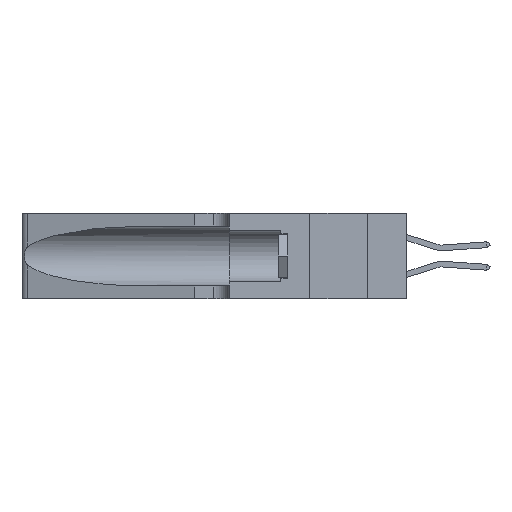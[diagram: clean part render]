
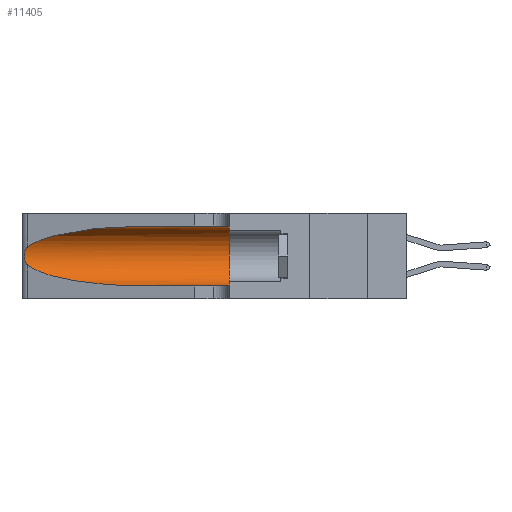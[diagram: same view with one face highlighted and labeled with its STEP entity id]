
A CAD part, left-side view. The second image highlights one B-rep face of the part: STEP entity #11405.
In plain terms, the highlighted cylindrical face has radius 3.308 mm (diameter 6.617 mm), a partial arc.
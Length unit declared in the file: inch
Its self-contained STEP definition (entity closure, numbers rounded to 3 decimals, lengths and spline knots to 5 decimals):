
#397 = CARTESIAN_POINT ( 'NONE',  ( 0.25789, 1.23486, 0.15765 ) ) ;
#1251 = DIRECTION ( 'NONE',  ( 0., -1., 0. ) ) ;
#2952 = CYLINDRICAL_SURFACE ( 'NONE', #24174, 0.13025 ) ;
#3356 = EDGE_CURVE ( 'NONE', #25811, #12666, #20754, .T. ) ;
#3742 = ORIENTED_EDGE ( 'NONE', *, *, #9370, .T. ) ;
#4027 = CARTESIAN_POINT ( 'NONE',  ( 0.18966, 0.96281, 0.31525 ) ) ;
#4162 = ORIENTED_EDGE ( 'NONE', *, *, #6636, .F. ) ;
#4529 = VERTEX_POINT ( 'NONE', #6289 ) ;
#5120 = CARTESIAN_POINT ( 'NONE',  ( 0.26075, 1.23896, 0.178 ) ) ;
#5314 = CARTESIAN_POINT ( 'NONE',  ( 0.25856, 1.23593, 0.16098 ) ) ;
#5771 = CARTESIAN_POINT ( 'NONE',  ( 0.1305, 1.61858, 0.185 ) ) ;
#6289 = CARTESIAN_POINT ( 'NONE',  ( 0.1305, 0.35, 0.05475 ) ) ;
#6322 = CARTESIAN_POINT ( 'NONE',  ( 0.2373, 1.15595, 0.28018 ) ) ;
#6623 = CARTESIAN_POINT ( 'NONE',  ( 0.25487, 1.22718, 0.22369 ) ) ;
#6636 = EDGE_CURVE ( 'NONE', #12883, #4529, #18485, .T. ) ;
#6882 = ORIENTED_EDGE ( 'NONE', *, *, #22389, .T. ) ;
#7833 = CARTESIAN_POINT ( 'NONE',  ( 0.25487, 1.22718, 0.14631 ) ) ;
#7922 = CARTESIAN_POINT ( 'NONE',  ( 0.1305, 1.61858, 0.05475 ) ) ;
#8382 = ORIENTED_EDGE ( 'NONE', *, *, #3356, .T. ) ;
#8412 = VECTOR ( 'NONE', #28521, 39.37008 ) ;
#8670 = CARTESIAN_POINT ( 'NONE',  ( 0.1305, 0.35, 0.31525 ) ) ;
#9370 = EDGE_CURVE ( 'NONE', #22631, #17043, #26556, .T. ) ;
#9446 = DIRECTION ( 'NONE',  ( 0., -1., 0. ) ) ;
#9896 = CARTESIAN_POINT ( 'NONE',  ( 0.25639, 1.23186, 0.15144 ) ) ;
#11096 = DIRECTION ( 'NONE',  ( 0., 0., 1. ) ) ;
#11405 = ADVANCED_FACE ( 'NONE', ( #11924 ), #2952, .F. ) ;
#11717 = CARTESIAN_POINT ( 'NONE',  ( 0.1305, 0.72297, 0.05475 ) ) ;
#11924 = FACE_OUTER_BOUND ( 'NONE', #18745, .T. ) ;
#12104 = CARTESIAN_POINT ( 'NONE',  ( 0.25555, 1.22994, 0.2215 ) ) ;
#12279 = ORIENTED_EDGE ( 'NONE', *, *, #28177, .F. ) ;
#12666 = VERTEX_POINT ( 'NONE', #18245 ) ;
#12883 = VERTEX_POINT ( 'NONE', #8670 ) ;
#13277 = B_SPLINE_CURVE_WITH_KNOTS ( 'NONE', 3,
 ( #14504, #12104, #23615, #27709, #18791, #14099, #18982, #5120, #14199, #5314, #397, #9896, #21247, #19078 ),
 .UNSPECIFIED., .F., .F.,
 ( 4, 2, 2, 2, 2, 2, 4 ),
 ( 0., 0.00027, 0.00053, 0.00107, 0.0016, 0.00187, 0.00214 ),
 .UNSPECIFIED. ) ;
#14099 = CARTESIAN_POINT ( 'NONE',  ( 0.26018, 1.23835, 0.19895 ) ) ;
#14199 = CARTESIAN_POINT ( 'NONE',  ( 0.26017, 1.23833, 0.17102 ) ) ;
#14233 = ORIENTED_EDGE ( 'NONE', *, *, #18139, .T. ) ;
#14504 = CARTESIAN_POINT ( 'NONE',  ( 0.25487, 1.22718, 0.22369 ) ) ;
#15575 = LINE ( 'NONE', #7922, #8412 ) ;
#15642 = CARTESIAN_POINT ( 'NONE',  ( 0.2373, 1.15595, 0.08982 ) ) ;
#17043 = VERTEX_POINT ( 'NONE', #28940 ) ;
#17242 = DIRECTION ( 'NONE',  ( 0., 0., -1. ) ) ;
#18139 = EDGE_CURVE ( 'NONE', #17043, #25811, #13277, .T. ) ;
#18245 = CARTESIAN_POINT ( 'NONE',  ( 0.1305, 0.72297, 0.05475 ) ) ;
#18485 = CIRCLE ( 'NONE', #19364, 0.13025 ) ;
#18745 = EDGE_LOOP ( 'NONE', ( #3742, #14233, #8382, #6882, #4162, #12279 ) ) ;
#18791 = CARTESIAN_POINT ( 'NONE',  ( 0.25854, 1.2359, 0.20912 ) ) ;
#18982 = CARTESIAN_POINT ( 'NONE',  ( 0.26075, 1.23896, 0.19203 ) ) ;
#19078 = CARTESIAN_POINT ( 'NONE',  ( 0.25487, 1.22718, 0.14631 ) ) ;
#19364 = AXIS2_PLACEMENT_3D ( 'NONE', #24706, #22613, #11096 ) ;
#19574 = VECTOR ( 'NONE', #9446, 39.37008 ) ;
#20109 = CARTESIAN_POINT ( 'NONE',  ( 0.1305, 0.72297, 0.31525 ) ) ;
#20700 = CARTESIAN_POINT ( 'NONE',  ( 0.18966, 0.96281, 0.05475 ) ) ;
#20754 =( BOUNDED_CURVE ( )  B_SPLINE_CURVE ( 3, ( #24887, #15642, #20700, #11717 ),
 .UNSPECIFIED., .F., .F. ) 
 B_SPLINE_CURVE_WITH_KNOTS ( ( 4, 4 ),
 ( 3.44316, 4.71239 ),
 .UNSPECIFIED. ) 
 CURVE ( )  GEOMETRIC_REPRESENTATION_ITEM ( )  RATIONAL_B_SPLINE_CURVE ( ( 1., 0.87, 0.87, 1. ) ) 
 REPRESENTATION_ITEM ( '' )  );
#21247 = CARTESIAN_POINT ( 'NONE',  ( 0.25555, 1.22993, 0.14849 ) ) ;
#22389 = EDGE_CURVE ( 'NONE', #12666, #4529, #15575, .T. ) ;
#22613 = DIRECTION ( 'NONE',  ( 0., 1., 0. ) ) ;
#22631 = VERTEX_POINT ( 'NONE', #20109 ) ;
#23279 = CARTESIAN_POINT ( 'NONE',  ( 0.1305, 1.61858, 0.31525 ) ) ;
#23615 = CARTESIAN_POINT ( 'NONE',  ( 0.25639, 1.23184, 0.21858 ) ) ;
#24174 = AXIS2_PLACEMENT_3D ( 'NONE', #5771, #1251, #17242 ) ;
#24706 = CARTESIAN_POINT ( 'NONE',  ( 0.1305, 0.35, 0.185 ) ) ;
#24887 = CARTESIAN_POINT ( 'NONE',  ( 0.25487, 1.22718, 0.14631 ) ) ;
#25811 = VERTEX_POINT ( 'NONE', #7833 ) ;
#26556 =( BOUNDED_CURVE ( )  B_SPLINE_CURVE ( 3, ( #28899, #4027, #6322, #6623 ),
 .UNSPECIFIED., .F., .F. ) 
 B_SPLINE_CURVE_WITH_KNOTS ( ( 4, 4 ),
 ( 1.5708, 2.84003 ),
 .UNSPECIFIED. ) 
 CURVE ( )  GEOMETRIC_REPRESENTATION_ITEM ( )  RATIONAL_B_SPLINE_CURVE ( ( 1., 0.87, 0.87, 1. ) ) 
 REPRESENTATION_ITEM ( '' )  );
#27709 = CARTESIAN_POINT ( 'NONE',  ( 0.25787, 1.23484, 0.2124 ) ) ;
#28177 = EDGE_CURVE ( 'NONE', #22631, #12883, #29154, .T. ) ;
#28521 = DIRECTION ( 'NONE',  ( 0., -1., 0. ) ) ;
#28899 = CARTESIAN_POINT ( 'NONE',  ( 0.1305, 0.72297, 0.31525 ) ) ;
#28940 = CARTESIAN_POINT ( 'NONE',  ( 0.25487, 1.22718, 0.22369 ) ) ;
#29154 = LINE ( 'NONE', #23279, #19574 ) ;
